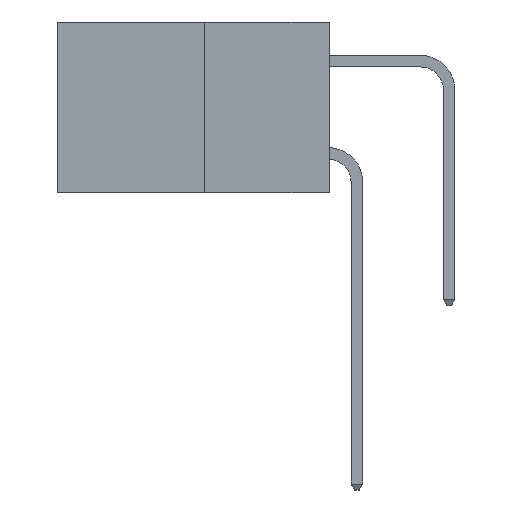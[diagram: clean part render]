
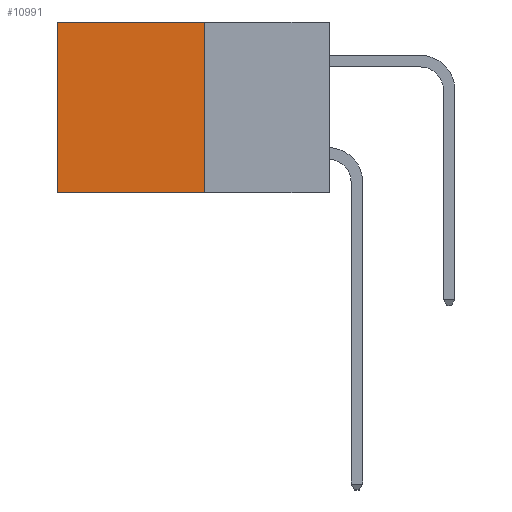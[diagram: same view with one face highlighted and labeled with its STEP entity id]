
A CAD part, left-side view. The second image highlights one B-rep face of the part: STEP entity #10991.
In plain terms, the highlighted planar face has unit normal (-1, 0, 0).
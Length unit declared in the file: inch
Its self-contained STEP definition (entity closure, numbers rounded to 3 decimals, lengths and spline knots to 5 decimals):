
#369 = DIRECTION ( 'NONE',  ( 0., 0., -1. ) ) ;
#642 = CARTESIAN_POINT ( 'NONE',  ( 0.277, 0.27, -0.37 ) ) ;
#818 = EDGE_CURVE ( 'NONE', #9888, #8095, #4796, .T. ) ;
#823 = CARTESIAN_POINT ( 'NONE',  ( 0.277, 0.27, -0.37 ) ) ;
#971 = ORIENTED_EDGE ( 'NONE', *, *, #818, .T. ) ;
#1028 = FACE_OUTER_BOUND ( 'NONE', #9540, .T. ) ;
#1053 = CARTESIAN_POINT ( 'NONE',  ( 0.277, 0.27, 0. ) ) ;
#1248 = EDGE_CURVE ( 'NONE', #4992, #8095, #14320, .T. ) ;
#1259 = ORIENTED_EDGE ( 'NONE', *, *, #4135, .T. ) ;
#1457 = VERTEX_POINT ( 'NONE', #1053 ) ;
#2767 = DIRECTION ( 'NONE',  ( 0., 1., 0. ) ) ;
#3215 = VECTOR ( 'NONE', #13775, 39.37008 ) ;
#3578 = ORIENTED_EDGE ( 'NONE', *, *, #17119, .F. ) ;
#3954 = DIRECTION ( 'NONE',  ( 0., 1., 0. ) ) ;
#4022 = CARTESIAN_POINT ( 'NONE',  ( 0.277, 0.27, 0. ) ) ;
#4135 = EDGE_CURVE ( 'NONE', #1457, #9888, #5660, .T. ) ;
#4796 = LINE ( 'NONE', #6389, #8580 ) ;
#4992 = VERTEX_POINT ( 'NONE', #11680 ) ;
#5660 = LINE ( 'NONE', #4022, #18817 ) ;
#5687 = DIRECTION ( 'NONE',  ( 0., 0., -1. ) ) ;
#6306 = VECTOR ( 'NONE', #2767, 39.37008 ) ;
#6357 = ORIENTED_EDGE ( 'NONE', *, *, #1248, .F. ) ;
#6389 = CARTESIAN_POINT ( 'NONE',  ( 0.277, 0.59, -0.37 ) ) ;
#7995 = AXIS2_PLACEMENT_3D ( 'NONE', #17987, #10165, #369 ) ;
#8095 = VERTEX_POINT ( 'NONE', #16792 ) ;
#8519 = PLANE ( 'NONE',  #7995 ) ;
#8580 = VECTOR ( 'NONE', #5687, 39.37008 ) ;
#9540 = EDGE_LOOP ( 'NONE', ( #971, #6357, #3578, #1259 ) ) ;
#9888 = VERTEX_POINT ( 'NONE', #14014 ) ;
#10165 = DIRECTION ( 'NONE',  ( 1., 0., 0. ) ) ;
#10991 = ADVANCED_FACE ( 'NONE', ( #1028 ), #8519, .F. ) ;
#11680 = CARTESIAN_POINT ( 'NONE',  ( 0.277, 0.27, -0.37 ) ) ;
#11865 = LINE ( 'NONE', #823, #3215 ) ;
#13775 = DIRECTION ( 'NONE',  ( 0., 0., -1. ) ) ;
#14014 = CARTESIAN_POINT ( 'NONE',  ( 0.277, 0.59, 0. ) ) ;
#14320 = LINE ( 'NONE', #642, #6306 ) ;
#16792 = CARTESIAN_POINT ( 'NONE',  ( 0.277, 0.59, -0.37 ) ) ;
#17119 = EDGE_CURVE ( 'NONE', #1457, #4992, #11865, .T. ) ;
#17987 = CARTESIAN_POINT ( 'NONE',  ( 0.277, 0.27, -0.37 ) ) ;
#18817 = VECTOR ( 'NONE', #3954, 39.37008 ) ;
